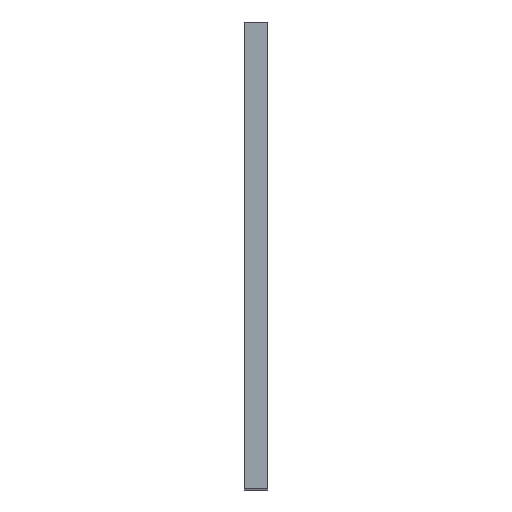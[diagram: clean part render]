
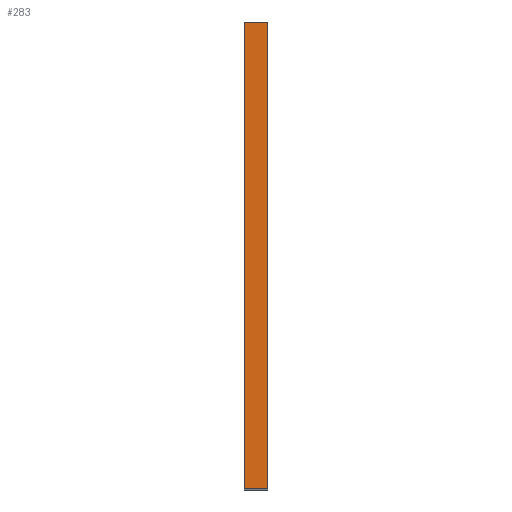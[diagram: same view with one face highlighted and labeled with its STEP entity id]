
A CAD part, top view. The second image highlights one B-rep face of the part: STEP entity #283.
In plain terms, the highlighted planar face has unit normal (0, 0, 1).
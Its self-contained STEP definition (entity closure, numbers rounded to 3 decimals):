
#20 = CARTESIAN_POINT ( 'NONE',  ( 4.375, -2.613, 34.061 ) ) ;
#73 = ORIENTED_EDGE ( 'NONE', *, *, #888, .F. ) ;
#105 = CARTESIAN_POINT ( 'NONE',  ( 0.625, -44.626, 34.061 ) ) ;
#130 = VERTEX_POINT ( 'NONE', #295 ) ;
#146 = DIRECTION ( 'NONE',  ( -1., 0., 0. ) ) ;
#151 = CARTESIAN_POINT ( 'NONE',  ( 4.375, -44.626, 34.061 ) ) ;
#176 = DIRECTION ( 'NONE',  ( 0., -1., 0. ) ) ;
#203 = CARTESIAN_POINT ( 'NONE',  ( 0.625, -2.613, 34.061 ) ) ;
#217 = EDGE_CURVE ( 'NONE', #380, #277, #817, .T. ) ;
#277 = VERTEX_POINT ( 'NONE', #105 ) ;
#283 = ADVANCED_FACE ( 'NONE', ( #792 ), #867, .F. ) ;
#295 = CARTESIAN_POINT ( 'NONE',  ( 4.375, -44.626, 34.061 ) ) ;
#336 = ORIENTED_EDGE ( 'NONE', *, *, #539, .F. ) ;
#341 = AXIS2_PLACEMENT_3D ( 'NONE', #20, #864, #860 ) ;
#369 = EDGE_LOOP ( 'NONE', ( #383, #73, #336, #487 ) ) ;
#380 = VERTEX_POINT ( 'NONE', #612 ) ;
#383 = ORIENTED_EDGE ( 'NONE', *, *, #217, .T. ) ;
#416 = EDGE_CURVE ( 'NONE', #451, #380, #675, .T. ) ;
#451 = VERTEX_POINT ( 'NONE', #604 ) ;
#487 = ORIENTED_EDGE ( 'NONE', *, *, #416, .T. ) ;
#518 = CARTESIAN_POINT ( 'NONE',  ( 4.375, -2.613, 34.061 ) ) ;
#520 = LINE ( 'NONE', #151, #522 ) ;
#522 = VECTOR ( 'NONE', #146, 1000. ) ;
#539 = EDGE_CURVE ( 'NONE', #451, #130, #641, .T. ) ;
#547 = DIRECTION ( 'NONE',  ( 0., -1., 0. ) ) ;
#583 = DIRECTION ( 'NONE',  ( -1., 0., 0. ) ) ;
#587 = CARTESIAN_POINT ( 'NONE',  ( 4.375, 28.499, 34.061 ) ) ;
#604 = CARTESIAN_POINT ( 'NONE',  ( 4.375, 28.499, 34.061 ) ) ;
#612 = CARTESIAN_POINT ( 'NONE',  ( 0.625, 28.499, 34.061 ) ) ;
#638 = VECTOR ( 'NONE', #547, 1000. ) ;
#641 = LINE ( 'NONE', #518, #638 ) ;
#663 = VECTOR ( 'NONE', #583, 1000. ) ;
#675 = LINE ( 'NONE', #587, #663 ) ;
#792 = FACE_OUTER_BOUND ( 'NONE', #369, .T. ) ;
#804 = VECTOR ( 'NONE', #176, 1000. ) ;
#817 = LINE ( 'NONE', #203, #804 ) ;
#860 = DIRECTION ( 'NONE',  ( 0., 1., 0. ) ) ;
#864 = DIRECTION ( 'NONE',  ( 0., 0., -1. ) ) ;
#867 = PLANE ( 'NONE',  #341 ) ;
#888 = EDGE_CURVE ( 'NONE', #130, #277, #520, .T. ) ;
